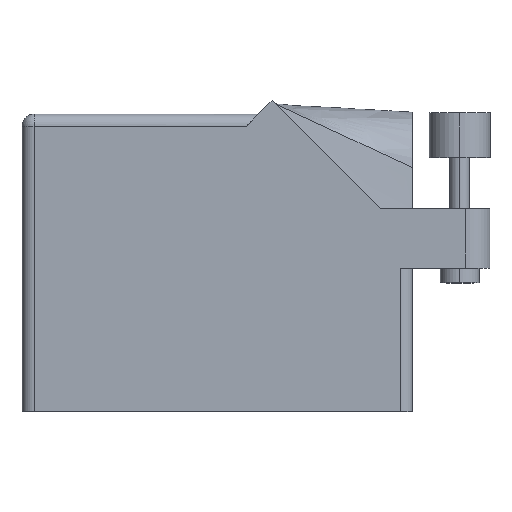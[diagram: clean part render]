
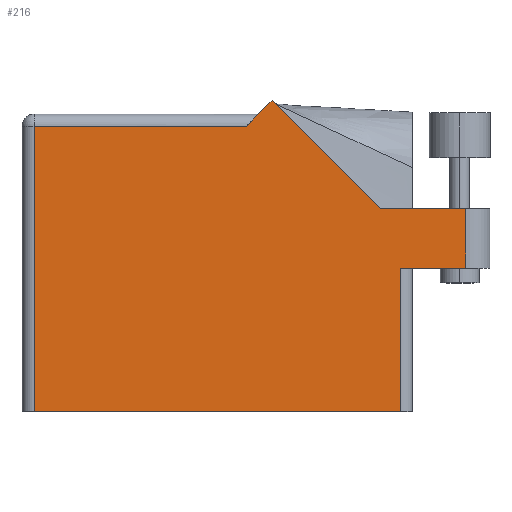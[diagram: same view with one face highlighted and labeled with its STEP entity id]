
A CAD part, top view. The second image highlights one B-rep face of the part: STEP entity #216.
In plain terms, the highlighted planar face has unit normal (0, 0, 1).
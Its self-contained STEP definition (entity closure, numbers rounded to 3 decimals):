
#12 = EDGE_CURVE ( 'NONE', #2353, #1208, #2158, .T. ) ;
#44 = DIRECTION ( 'NONE',  ( 1., 0., 0. ) ) ;
#57 = EDGE_CURVE ( 'NONE', #1521, #2107, #799, .T. ) ;
#58 = CARTESIAN_POINT ( 'NONE',  ( 0., 37.287, 0. ) ) ;
#61 = EDGE_CURVE ( 'NONE', #2107, #2353, #616, .T. ) ;
#74 = VECTOR ( 'NONE', #947, 1000. ) ;
#95 = VECTOR ( 'NONE', #1417, 1000. ) ;
#107 = VECTOR ( 'NONE', #936, 1000. ) ;
#136 = VERTEX_POINT ( 'NONE', #1270 ) ;
#216 = ADVANCED_FACE ( 'NONE', ( #685 ), #1093, .F. ) ;
#223 = AXIS2_PLACEMENT_3D ( 'NONE', #878, #498, #1462 ) ;
#238 = CARTESIAN_POINT ( 'NONE',  ( 51.054, 18.72, 0. ) ) ;
#294 = DIRECTION ( 'NONE',  ( 1., 0., 0. ) ) ;
#301 = VERTEX_POINT ( 'NONE', #2305 ) ;
#341 = ORIENTED_EDGE ( 'NONE', *, *, #61, .T. ) ;
#360 = LINE ( 'NONE', #2295, #74 ) ;
#365 = ORIENTED_EDGE ( 'NONE', *, *, #1225, .T. ) ;
#393 = ORIENTED_EDGE ( 'NONE', *, *, #12, .T. ) ;
#498 = DIRECTION ( 'NONE',  ( 0., 0., -1. ) ) ;
#505 = VECTOR ( 'NONE', #1802, 1000. ) ;
#511 = EDGE_CURVE ( 'NONE', #1208, #1102, #1592, .T. ) ;
#560 = CARTESIAN_POINT ( 'NONE',  ( 58.039, 18.72, 0. ) ) ;
#576 = VERTEX_POINT ( 'NONE', #729 ) ;
#616 = LINE ( 'NONE', #238, #2077 ) ;
#631 = CARTESIAN_POINT ( 'NONE',  ( 46.848, 26.518, 0. ) ) ;
#652 = CARTESIAN_POINT ( 'NONE',  ( 61.214, 26.518, 0. ) ) ;
#676 = DIRECTION ( 'NONE',  ( 0., -1., 0. ) ) ;
#685 = FACE_OUTER_BOUND ( 'NONE', #1486, .T. ) ;
#729 = CARTESIAN_POINT ( 'NONE',  ( 32.708, 40.658, 0. ) ) ;
#781 = EDGE_CURVE ( 'NONE', #1241, #1521, #1289, .T. ) ;
#799 = LINE ( 'NONE', #1200, #1479 ) ;
#878 = CARTESIAN_POINT ( 'NONE',  ( 0., 38.862, 0. ) ) ;
#936 = DIRECTION ( 'NONE',  ( -0.707, 0.707, 0. ) ) ;
#947 = DIRECTION ( 'NONE',  ( -0.707, -0.707, 0. ) ) ;
#990 = VECTOR ( 'NONE', #294, 1000. ) ;
#1050 = CARTESIAN_POINT ( 'NONE',  ( 49.479, 18.72, 0. ) ) ;
#1056 = CARTESIAN_POINT ( 'NONE',  ( 1.575, 0., 0. ) ) ;
#1082 = CARTESIAN_POINT ( 'NONE',  ( 58.039, 26.518, 0. ) ) ;
#1093 = PLANE ( 'NONE',  #223 ) ;
#1102 = VERTEX_POINT ( 'NONE', #631 ) ;
#1163 = EDGE_CURVE ( 'NONE', #136, #301, #2336, .T. ) ;
#1200 = CARTESIAN_POINT ( 'NONE',  ( 49.479, 18.72, 0. ) ) ;
#1208 = VERTEX_POINT ( 'NONE', #1082 ) ;
#1225 = EDGE_CURVE ( 'NONE', #301, #1241, #1424, .T. ) ;
#1241 = VERTEX_POINT ( 'NONE', #1433 ) ;
#1249 = VECTOR ( 'NONE', #676, 1000. ) ;
#1257 = ORIENTED_EDGE ( 'NONE', *, *, #511, .T. ) ;
#1270 = CARTESIAN_POINT ( 'NONE',  ( 29.337, 37.287, 0. ) ) ;
#1289 = LINE ( 'NONE', #1818, #990 ) ;
#1368 = EDGE_CURVE ( 'NONE', #576, #136, #360, .T. ) ;
#1383 = DIRECTION ( 'NONE',  ( -1., 0., 0. ) ) ;
#1417 = DIRECTION ( 'NONE',  ( -1., 0., 0. ) ) ;
#1424 = LINE ( 'NONE', #1056, #1249 ) ;
#1433 = CARTESIAN_POINT ( 'NONE',  ( 1.575, 0., 0. ) ) ;
#1462 = DIRECTION ( 'NONE',  ( -1., 0., 0. ) ) ;
#1479 = VECTOR ( 'NONE', #2180, 1000. ) ;
#1486 = EDGE_LOOP ( 'NONE', ( #341, #393, #1257, #2480, #2109, #2324, #365, #2204, #1594 ) ) ;
#1511 = LINE ( 'NONE', #2063, #107 ) ;
#1521 = VERTEX_POINT ( 'NONE', #1570 ) ;
#1570 = CARTESIAN_POINT ( 'NONE',  ( 49.479, 0., 0. ) ) ;
#1592 = LINE ( 'NONE', #652, #95 ) ;
#1594 = ORIENTED_EDGE ( 'NONE', *, *, #57, .T. ) ;
#1653 = VECTOR ( 'NONE', #1383, 1000. ) ;
#1802 = DIRECTION ( 'NONE',  ( 0., 1., 0. ) ) ;
#1818 = CARTESIAN_POINT ( 'NONE',  ( 0., 0., 0. ) ) ;
#1948 = CARTESIAN_POINT ( 'NONE',  ( 58.039, 26.518, 0. ) ) ;
#2063 = CARTESIAN_POINT ( 'NONE',  ( 46.848, 26.518, 0. ) ) ;
#2077 = VECTOR ( 'NONE', #44, 1000. ) ;
#2107 = VERTEX_POINT ( 'NONE', #1050 ) ;
#2109 = ORIENTED_EDGE ( 'NONE', *, *, #1368, .T. ) ;
#2158 = LINE ( 'NONE', #1948, #505 ) ;
#2180 = DIRECTION ( 'NONE',  ( 0., 1., 0. ) ) ;
#2204 = ORIENTED_EDGE ( 'NONE', *, *, #781, .T. ) ;
#2295 = CARTESIAN_POINT ( 'NONE',  ( 30.912, 38.862, 0. ) ) ;
#2303 = EDGE_CURVE ( 'NONE', #1102, #576, #1511, .T. ) ;
#2305 = CARTESIAN_POINT ( 'NONE',  ( 1.575, 37.287, 0. ) ) ;
#2324 = ORIENTED_EDGE ( 'NONE', *, *, #1163, .T. ) ;
#2336 = LINE ( 'NONE', #58, #1653 ) ;
#2353 = VERTEX_POINT ( 'NONE', #560 ) ;
#2480 = ORIENTED_EDGE ( 'NONE', *, *, #2303, .T. ) ;
